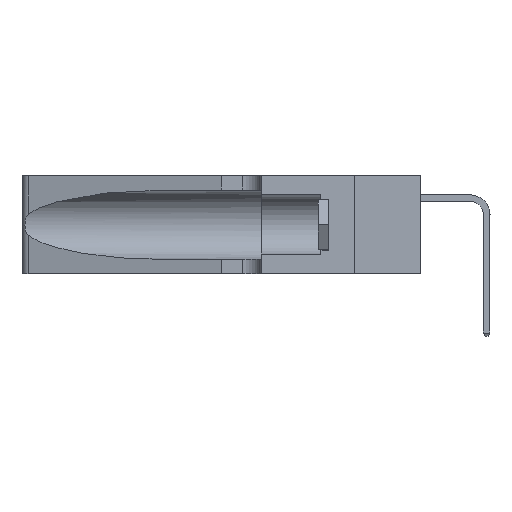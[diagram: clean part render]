
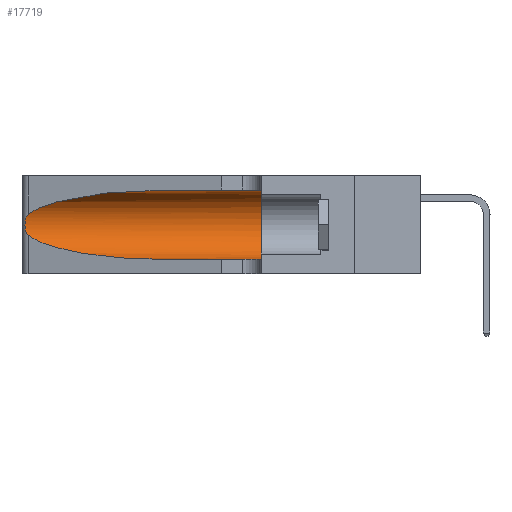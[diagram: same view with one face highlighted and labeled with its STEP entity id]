
A CAD part, left-side view. The second image highlights one B-rep face of the part: STEP entity #17719.
In plain terms, the highlighted cylindrical face has radius 3.308 mm (diameter 6.617 mm), a partial arc.
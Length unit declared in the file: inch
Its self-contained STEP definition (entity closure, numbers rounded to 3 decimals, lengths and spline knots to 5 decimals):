
#609 = VERTEX_POINT ( 'NONE', #35062 ) ;
#1382 = VERTEX_POINT ( 'NONE', #28511 ) ;
#1587 = CARTESIAN_POINT ( 'NONE',  ( 0.25787, 1.23484, 0.2124 ) ) ;
#2035 = B_SPLINE_CURVE_WITH_KNOTS ( 'NONE', 3,
 ( #37171, #33604, #23025, #1587, #26626, #5196, #30172, #8826, #33754, #12439, #37321, #16028, #40886, #19617 ),
 .UNSPECIFIED., .F., .F.,
 ( 4, 2, 2, 2, 2, 2, 4 ),
 ( 0., 0.00027, 0.00053, 0.00107, 0.0016, 0.00187, 0.00214 ),
 .UNSPECIFIED. ) ;
#2101 = CARTESIAN_POINT ( 'NONE',  ( 0.1305, 0.35, 0.31525 ) ) ;
#2398 = ORIENTED_EDGE ( 'NONE', *, *, #12032, .T. ) ;
#5141 = LINE ( 'NONE', #21402, #40830 ) ;
#5196 = CARTESIAN_POINT ( 'NONE',  ( 0.26018, 1.23835, 0.19895 ) ) ;
#6692 = CARTESIAN_POINT ( 'NONE',  ( 0.1305, 0.72297, 0.05475 ) ) ;
#6908 = DIRECTION ( 'NONE',  ( 0., -1., 0. ) ) ;
#6975 = CARTESIAN_POINT ( 'NONE',  ( 0.25487, 1.22718, 0.14631 ) ) ;
#7008 = EDGE_CURVE ( 'NONE', #21079, #9564, #45706, .T. ) ;
#7656 = AXIS2_PLACEMENT_3D ( 'NONE', #18311, #43116, #21878 ) ;
#7869 = DIRECTION ( 'NONE',  ( 0., 0., -1. ) ) ;
#8052 = EDGE_LOOP ( 'NONE', ( #8514, #9188, #20807, #2398, #25632, #44545 ) ) ;
#8514 = ORIENTED_EDGE ( 'NONE', *, *, #19980, .T. ) ;
#8826 = CARTESIAN_POINT ( 'NONE',  ( 0.26075, 1.23896, 0.178 ) ) ;
#9188 = ORIENTED_EDGE ( 'NONE', *, *, #25951, .T. ) ;
#9564 = VERTEX_POINT ( 'NONE', #2101 ) ;
#10333 = CARTESIAN_POINT ( 'NONE',  ( 0.2373, 1.15595, 0.28018 ) ) ;
#11328 = CYLINDRICAL_SURFACE ( 'NONE', #24800, 0.13025 ) ;
#12032 = EDGE_CURVE ( 'NONE', #35248, #609, #5141, .T. ) ;
#12439 = CARTESIAN_POINT ( 'NONE',  ( 0.25856, 1.23593, 0.16098 ) ) ;
#16028 = CARTESIAN_POINT ( 'NONE',  ( 0.25639, 1.23186, 0.15144 ) ) ;
#17719 = ADVANCED_FACE ( 'NONE', ( #39707 ), #11328, .F. ) ;
#17926 = CARTESIAN_POINT ( 'NONE',  ( 0.18966, 0.96281, 0.05475 ) ) ;
#18311 = CARTESIAN_POINT ( 'NONE',  ( 0.1305, 0.35, 0.185 ) ) ;
#19617 = CARTESIAN_POINT ( 'NONE',  ( 0.25487, 1.22718, 0.14631 ) ) ;
#19980 = EDGE_CURVE ( 'NONE', #21079, #1382, #37177, .T. ) ;
#20807 = ORIENTED_EDGE ( 'NONE', *, *, #39309, .T. ) ;
#21079 = VERTEX_POINT ( 'NONE', #28821 ) ;
#21350 = CARTESIAN_POINT ( 'NONE',  ( 0.2373, 1.15595, 0.08982 ) ) ;
#21402 = CARTESIAN_POINT ( 'NONE',  ( 0.1305, 1.61858, 0.05475 ) ) ;
#21878 = DIRECTION ( 'NONE',  ( 0., 0., 1. ) ) ;
#23025 = CARTESIAN_POINT ( 'NONE',  ( 0.25639, 1.23184, 0.21858 ) ) ;
#24800 = AXIS2_PLACEMENT_3D ( 'NONE', #32802, #36379, #7869 ) ;
#25632 = ORIENTED_EDGE ( 'NONE', *, *, #41990, .F. ) ;
#25951 = EDGE_CURVE ( 'NONE', #1382, #34881, #2035, .T. ) ;
#26626 = CARTESIAN_POINT ( 'NONE',  ( 0.25854, 1.2359, 0.20912 ) ) ;
#27998 = CARTESIAN_POINT ( 'NONE',  ( 0.1305, 0.72297, 0.31525 ) ) ;
#28511 = CARTESIAN_POINT ( 'NONE',  ( 0.25487, 1.22718, 0.22369 ) ) ;
#28821 = CARTESIAN_POINT ( 'NONE',  ( 0.1305, 0.72297, 0.31525 ) ) ;
#30172 = CARTESIAN_POINT ( 'NONE',  ( 0.26075, 1.23896, 0.19203 ) ) ;
#31801 = CIRCLE ( 'NONE', #7656, 0.13025 ) ;
#32802 = CARTESIAN_POINT ( 'NONE',  ( 0.1305, 1.61858, 0.185 ) ) ;
#33604 = CARTESIAN_POINT ( 'NONE',  ( 0.25555, 1.22994, 0.2215 ) ) ;
#33754 = CARTESIAN_POINT ( 'NONE',  ( 0.26017, 1.23833, 0.17102 ) ) ;
#34881 = VERTEX_POINT ( 'NONE', #36909 ) ;
#35062 = CARTESIAN_POINT ( 'NONE',  ( 0.1305, 0.35, 0.05475 ) ) ;
#35248 = VERTEX_POINT ( 'NONE', #6692 ) ;
#35256 = CARTESIAN_POINT ( 'NONE',  ( 0.25487, 1.22718, 0.22369 ) ) ;
#35406 = CARTESIAN_POINT ( 'NONE',  ( 0.1305, 1.61858, 0.31525 ) ) ;
#36379 = DIRECTION ( 'NONE',  ( 0., -1., 0. ) ) ;
#36909 = CARTESIAN_POINT ( 'NONE',  ( 0.25487, 1.22718, 0.14631 ) ) ;
#37171 = CARTESIAN_POINT ( 'NONE',  ( 0.25487, 1.22718, 0.22369 ) ) ;
#37177 =( BOUNDED_CURVE ( )  B_SPLINE_CURVE ( 3, ( #27998, #45802, #10333, #35256 ),
 .UNSPECIFIED., .F., .F. ) 
 B_SPLINE_CURVE_WITH_KNOTS ( ( 4, 4 ),
 ( 1.5708, 2.84003 ),
 .UNSPECIFIED. ) 
 CURVE ( )  GEOMETRIC_REPRESENTATION_ITEM ( )  RATIONAL_B_SPLINE_CURVE ( ( 1., 0.87, 0.87, 1. ) ) 
 REPRESENTATION_ITEM ( '' )  );
#37321 = CARTESIAN_POINT ( 'NONE',  ( 0.25789, 1.23486, 0.15765 ) ) ;
#39100 = DIRECTION ( 'NONE',  ( 0., -1., 0. ) ) ;
#39309 = EDGE_CURVE ( 'NONE', #34881, #35248, #40578, .T. ) ;
#39707 = FACE_OUTER_BOUND ( 'NONE', #8052, .T. ) ;
#40578 =( BOUNDED_CURVE ( )  B_SPLINE_CURVE ( 3, ( #6975, #21350, #17926, #42755 ),
 .UNSPECIFIED., .F., .F. ) 
 B_SPLINE_CURVE_WITH_KNOTS ( ( 4, 4 ),
 ( 3.44316, 4.71239 ),
 .UNSPECIFIED. ) 
 CURVE ( )  GEOMETRIC_REPRESENTATION_ITEM ( )  RATIONAL_B_SPLINE_CURVE ( ( 1., 0.87, 0.87, 1. ) ) 
 REPRESENTATION_ITEM ( '' )  );
#40830 = VECTOR ( 'NONE', #39100, 39.37008 ) ;
#40886 = CARTESIAN_POINT ( 'NONE',  ( 0.25555, 1.22993, 0.14849 ) ) ;
#41990 = EDGE_CURVE ( 'NONE', #9564, #609, #31801, .T. ) ;
#42755 = CARTESIAN_POINT ( 'NONE',  ( 0.1305, 0.72297, 0.05475 ) ) ;
#43116 = DIRECTION ( 'NONE',  ( 0., 1., 0. ) ) ;
#44545 = ORIENTED_EDGE ( 'NONE', *, *, #7008, .F. ) ;
#44595 = VECTOR ( 'NONE', #6908, 39.37008 ) ;
#45706 = LINE ( 'NONE', #35406, #44595 ) ;
#45802 = CARTESIAN_POINT ( 'NONE',  ( 0.18966, 0.96281, 0.31525 ) ) ;
